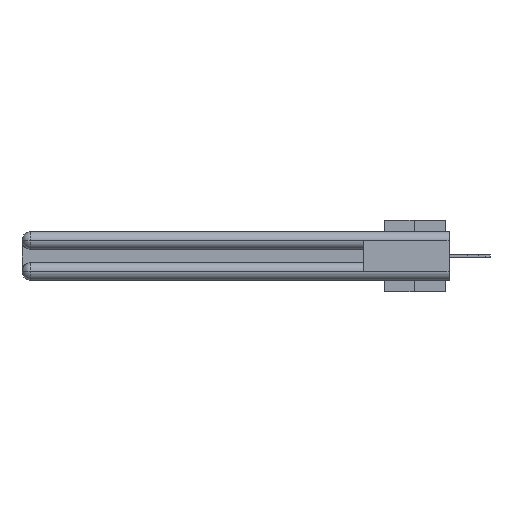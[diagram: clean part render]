
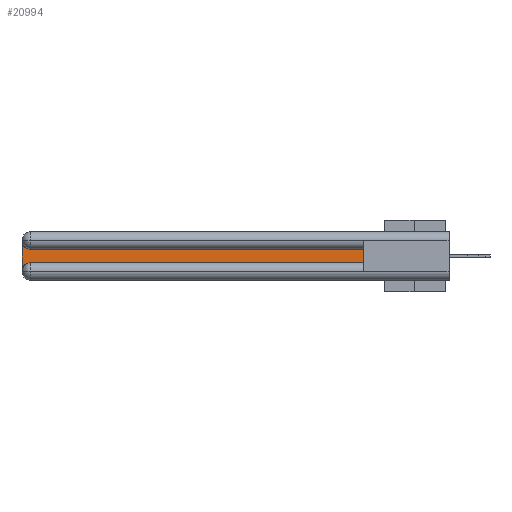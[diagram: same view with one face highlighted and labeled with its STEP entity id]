
A CAD part, left-side view. The second image highlights one B-rep face of the part: STEP entity #20994.
In plain terms, the highlighted planar face has unit normal (-1, 0, 0).
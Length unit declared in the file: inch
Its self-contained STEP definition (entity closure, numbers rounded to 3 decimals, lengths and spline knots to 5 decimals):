
#181 = ORIENTED_EDGE ( 'NONE', *, *, #6242, .T. ) ;
#398 = DIRECTION ( 'NONE',  ( 0., -1., 0. ) ) ;
#973 = CARTESIAN_POINT ( 'NONE',  ( 0.075, 2.94, -0.2775 ) ) ;
#1013 = PLANE ( 'NONE',  #22939 ) ;
#1246 = CARTESIAN_POINT ( 'NONE',  ( 0.075, 0.6, -0.1225 ) ) ;
#1267 = DIRECTION ( 'NONE',  ( 0., 0., -1. ) ) ;
#1896 = VERTEX_POINT ( 'NONE', #10003 ) ;
#2545 = CARTESIAN_POINT ( 'NONE',  ( 0.075, 2.94, -0.0625 ) ) ;
#3619 = CIRCLE ( 'NONE', #10891, 0.06 ) ;
#3663 = DIRECTION ( 'NONE',  ( 0., 0., -1. ) ) ;
#3701 = CARTESIAN_POINT ( 'NONE',  ( 0.075, 3., -0.2775 ) ) ;
#3707 = CARTESIAN_POINT ( 'NONE',  ( 0.075, 3., -0.1225 ) ) ;
#4087 = VERTEX_POINT ( 'NONE', #11117 ) ;
#5036 = ORIENTED_EDGE ( 'NONE', *, *, #30705, .T. ) ;
#5165 = DIRECTION ( 'NONE',  ( 0., 0., -1. ) ) ;
#5578 = CARTESIAN_POINT ( 'NONE',  ( 0.075, 0.6, -0.2175 ) ) ;
#5968 = CARTESIAN_POINT ( 'NONE',  ( 0.075, 2.94, -0.2175 ) ) ;
#6242 = EDGE_CURVE ( 'NONE', #18117, #15024, #32038, .T. ) ;
#6318 = DIRECTION ( 'NONE',  ( 0., 0., -1. ) ) ;
#6549 = DIRECTION ( 'NONE',  ( 0., 1., 0. ) ) ;
#6566 = CARTESIAN_POINT ( 'NONE',  ( 0.075, 3., -0.2175 ) ) ;
#6836 = VECTOR ( 'NONE', #398, 39.37008 ) ;
#8293 = LINE ( 'NONE', #1246, #26376 ) ;
#8477 = LINE ( 'NONE', #5578, #6836 ) ;
#10003 = CARTESIAN_POINT ( 'NONE',  ( 0.075, 0.6, -0.1225 ) ) ;
#10155 = EDGE_CURVE ( 'NONE', #15024, #20541, #8477, .T. ) ;
#10891 = AXIS2_PLACEMENT_3D ( 'NONE', #2545, #20968, #5165 ) ;
#11117 = CARTESIAN_POINT ( 'NONE',  ( 0.075, 3., -0.0625 ) ) ;
#11802 = LINE ( 'NONE', #6566, #25783 ) ;
#13530 = EDGE_CURVE ( 'NONE', #1896, #22279, #8293, .T. ) ;
#14374 = FACE_OUTER_BOUND ( 'NONE', #22951, .T. ) ;
#14550 = AXIS2_PLACEMENT_3D ( 'NONE', #973, #19404, #3663 ) ;
#15024 = VERTEX_POINT ( 'NONE', #5968 ) ;
#15756 = ORIENTED_EDGE ( 'NONE', *, *, #26547, .T. ) ;
#16309 = CARTESIAN_POINT ( 'NONE',  ( 0.075, 0.6, -0.2175 ) ) ;
#16743 = EDGE_CURVE ( 'NONE', #22279, #4087, #3619, .T. ) ;
#17033 = VECTOR ( 'NONE', #23018, 39.37008 ) ;
#18117 = VERTEX_POINT ( 'NONE', #3701 ) ;
#19360 = CARTESIAN_POINT ( 'NONE',  ( 0.075, 2.94, -0.1225 ) ) ;
#19404 = DIRECTION ( 'NONE',  ( 1., 0., 0. ) ) ;
#20361 = CARTESIAN_POINT ( 'NONE',  ( 0.075, 0.6, -0.2175 ) ) ;
#20541 = VERTEX_POINT ( 'NONE', #16309 ) ;
#20968 = DIRECTION ( 'NONE',  ( 1., 0., 0. ) ) ;
#20994 = ADVANCED_FACE ( 'NONE', ( #14374 ), #1013, .F. ) ;
#22114 = DIRECTION ( 'NONE',  ( 1., 0., 0. ) ) ;
#22279 = VERTEX_POINT ( 'NONE', #19360 ) ;
#22939 = AXIS2_PLACEMENT_3D ( 'NONE', #3707, #22114, #6318 ) ;
#22951 = EDGE_LOOP ( 'NONE', ( #26679, #31701, #15756, #181, #29682, #5036 ) ) ;
#23018 = DIRECTION ( 'NONE',  ( 0., 0., 1. ) ) ;
#25614 = LINE ( 'NONE', #20361, #17033 ) ;
#25783 = VECTOR ( 'NONE', #1267, 39.37008 ) ;
#26376 = VECTOR ( 'NONE', #6549, 39.37008 ) ;
#26547 = EDGE_CURVE ( 'NONE', #4087, #18117, #11802, .T. ) ;
#26679 = ORIENTED_EDGE ( 'NONE', *, *, #13530, .T. ) ;
#29682 = ORIENTED_EDGE ( 'NONE', *, *, #10155, .T. ) ;
#30705 = EDGE_CURVE ( 'NONE', #20541, #1896, #25614, .T. ) ;
#31701 = ORIENTED_EDGE ( 'NONE', *, *, #16743, .T. ) ;
#32038 = CIRCLE ( 'NONE', #14550, 0.06 ) ;
